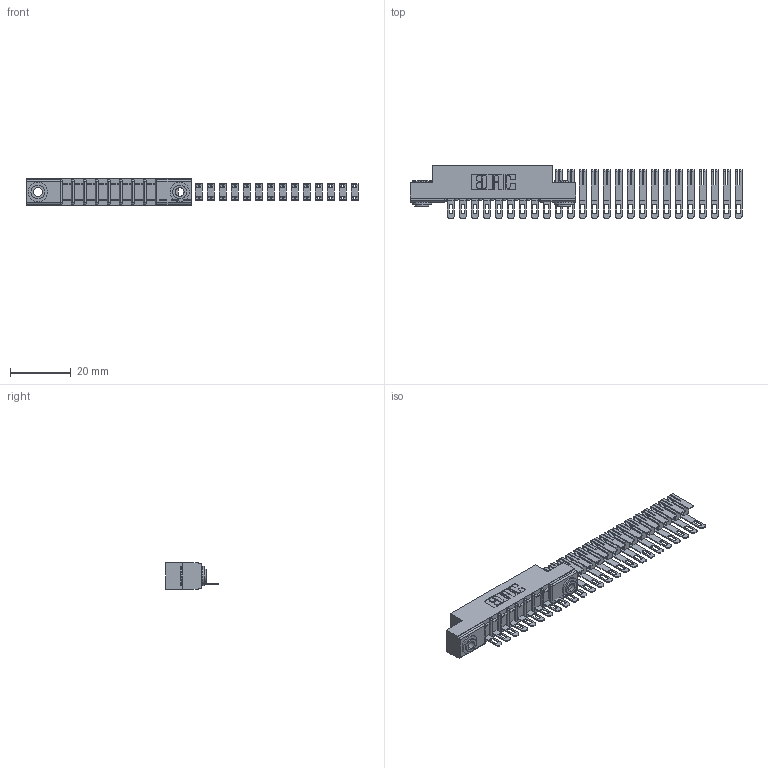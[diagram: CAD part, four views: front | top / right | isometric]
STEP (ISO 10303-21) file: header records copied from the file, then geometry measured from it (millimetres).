
FILE_DESCRIPTION (( 'STEP AP203' ), '1' );
FILE_NAME ('357-025-501-103.STEP', '2018-08-09T01:59:28', ( '' ), ( '' ), 'SwSTEP 2.0', 'SolidWorks 2016', '' );
FILE_SCHEMA (( 'CONFIG_CONTROL_DESIGN' ));
Length unit declared in the file: inch
Products named in the file (4): 307 Part_.156 Dia Mounting Holes; 307-290-002_501; 345-250-002_345-250-002-102; 357-025-501-103
Assembly tree (28 placements, depth 2):
  357-025-501-103
    307 Part_.156 Dia Mounting Holes
    307-290-002_501  x25
    345-250-002_345-250-002-102  x2
Bounding box: 109.72 x 17.42 x 8.71 mm (x, y, z)
Volume: 4119.6 mm3; surface area: 9993.5 mm2
Topology: 28 solids, 28 shells, 1739 faces, 5297 edges, 3502 vertices
Faces by surface type: plane 990, cylinder 723, sphere 18, cone 8
Entity records: 13453 total; most frequent: CARTESIAN_POINT 2166, DIRECTION 2157, ORIENTED_EDGE 2130, EDGE_CURVE 1065, VECTOR 787, LINE 787, VERTEX_POINT 694, AXIS2_PLACEMENT_3D 685
